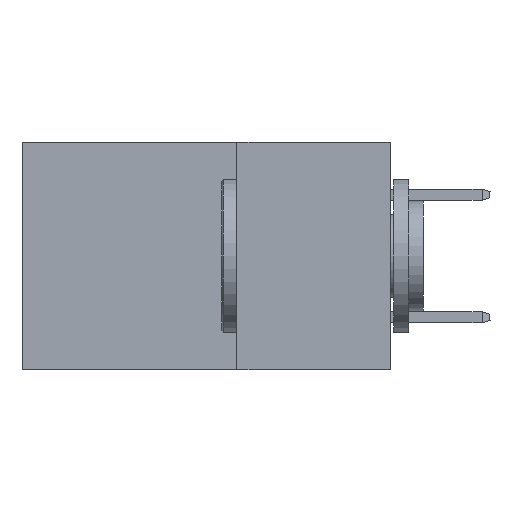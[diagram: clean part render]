
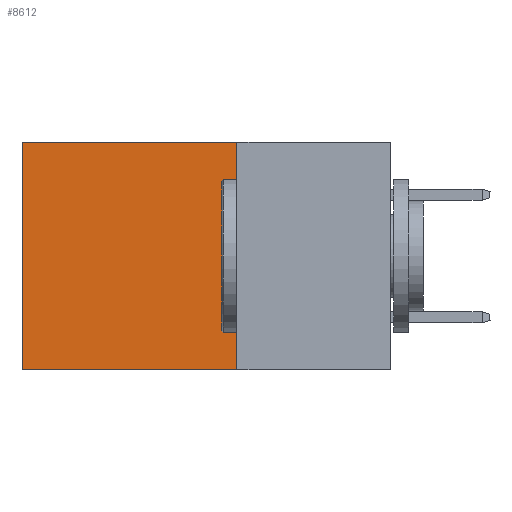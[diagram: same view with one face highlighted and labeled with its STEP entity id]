
A CAD part, left-side view. The second image highlights one B-rep face of the part: STEP entity #8612.
In plain terms, the highlighted planar face has unit normal (-1, 0, 0).
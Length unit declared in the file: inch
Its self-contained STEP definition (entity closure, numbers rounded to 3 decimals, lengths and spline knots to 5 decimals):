
#67 = LINE ( 'NONE', #2808, #5051 ) ;
#2176 = CARTESIAN_POINT ( 'NONE',  ( 0.2875, 0.25, -0.37 ) ) ;
#2190 = CARTESIAN_POINT ( 'NONE',  ( 0.2875, 0.6, -0.37 ) ) ;
#2635 = DIRECTION ( 'NONE',  ( 0., 1., 0. ) ) ;
#2808 = CARTESIAN_POINT ( 'NONE',  ( 0.2875, 0.25, -0.37 ) ) ;
#2813 = ORIENTED_EDGE ( 'NONE', *, *, #5675, .F. ) ;
#2932 = LINE ( 'NONE', #5680, #5210 ) ;
#3109 = VERTEX_POINT ( 'NONE', #6286 ) ;
#3697 = VERTEX_POINT ( 'NONE', #2176 ) ;
#3703 = VERTEX_POINT ( 'NONE', #2190 ) ;
#4503 = EDGE_CURVE ( 'NONE', #6395, #3109, #2932, .T. ) ;
#4619 = ORIENTED_EDGE ( 'NONE', *, *, #4503, .T. ) ;
#4740 = EDGE_CURVE ( 'NONE', #3697, #3703, #67, .T. ) ;
#4742 = VECTOR ( 'NONE', #9727, 39.37008 ) ;
#4793 = PLANE ( 'NONE',  #8762 ) ;
#4837 = CARTESIAN_POINT ( 'NONE',  ( 0.2875, 0.6, 0. ) ) ;
#5051 = VECTOR ( 'NONE', #2635, 39.37008 ) ;
#5210 = VECTOR ( 'NONE', #5615, 39.37008 ) ;
#5416 = CARTESIAN_POINT ( 'NONE',  ( 0.2875, 0.25, 0. ) ) ;
#5615 = DIRECTION ( 'NONE',  ( 0., 1., 0. ) ) ;
#5675 = EDGE_CURVE ( 'NONE', #6395, #3697, #7251, .T. ) ;
#5680 = CARTESIAN_POINT ( 'NONE',  ( 0.2875, 0.25, 0. ) ) ;
#6286 = CARTESIAN_POINT ( 'NONE',  ( 0.2875, 0.6, 0. ) ) ;
#6362 = ORIENTED_EDGE ( 'NONE', *, *, #4740, .F. ) ;
#6395 = VERTEX_POINT ( 'NONE', #8954 ) ;
#6670 = DIRECTION ( 'NONE',  ( 0., 0., -1. ) ) ;
#7091 = ORIENTED_EDGE ( 'NONE', *, *, #8641, .T. ) ;
#7251 = LINE ( 'NONE', #5416, #4742 ) ;
#8423 = LINE ( 'NONE', #4837, #10811 ) ;
#8612 = ADVANCED_FACE ( 'NONE', ( #11084 ), #4793, .F. ) ;
#8641 = EDGE_CURVE ( 'NONE', #3109, #3703, #8423, .T. ) ;
#8762 = AXIS2_PLACEMENT_3D ( 'NONE', #11209, #12095, #6670 ) ;
#8954 = CARTESIAN_POINT ( 'NONE',  ( 0.2875, 0.25, 0. ) ) ;
#9465 = DIRECTION ( 'NONE',  ( 0., 0., -1. ) ) ;
#9727 = DIRECTION ( 'NONE',  ( 0., 0., -1. ) ) ;
#10389 = EDGE_LOOP ( 'NONE', ( #7091, #6362, #2813, #4619 ) ) ;
#10811 = VECTOR ( 'NONE', #9465, 39.37008 ) ;
#11084 = FACE_OUTER_BOUND ( 'NONE', #10389, .T. ) ;
#11209 = CARTESIAN_POINT ( 'NONE',  ( 0.2875, 0.25, 0. ) ) ;
#12095 = DIRECTION ( 'NONE',  ( 1., 0., 0. ) ) ;
